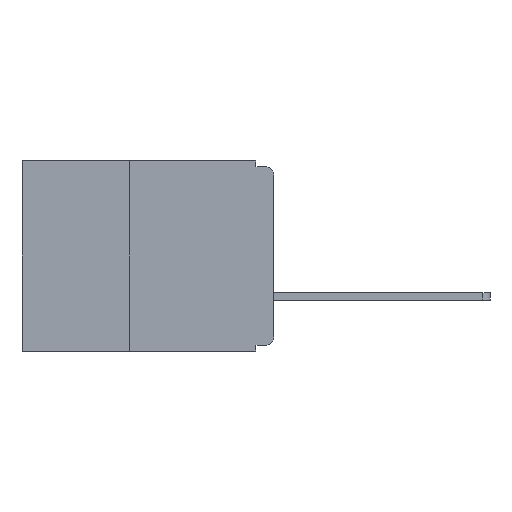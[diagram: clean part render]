
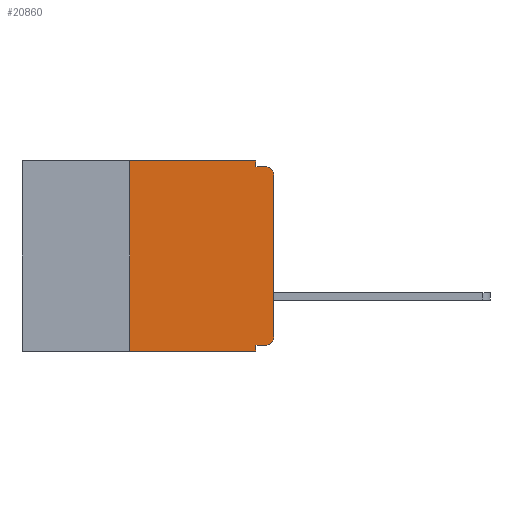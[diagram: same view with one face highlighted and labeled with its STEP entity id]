
A CAD part, left-side view. The second image highlights one B-rep face of the part: STEP entity #20860.
In plain terms, the highlighted planar face has unit normal (-1, 0, 0).
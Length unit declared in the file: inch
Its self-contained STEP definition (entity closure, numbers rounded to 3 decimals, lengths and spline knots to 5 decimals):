
#31 = CIRCLE ( 'NONE', #7282, 0.015 ) ;
#987 = VECTOR ( 'NONE', #13151, 39.37008 ) ;
#1114 = ORIENTED_EDGE ( 'NONE', *, *, #11044, .F. ) ;
#1676 = VECTOR ( 'NONE', #19482, 39.37008 ) ;
#2012 = CARTESIAN_POINT ( 'NONE',  ( 0., 0.437, 0. ) ) ;
#2545 = EDGE_CURVE ( 'NONE', #19357, #19807, #5549, .T. ) ;
#2697 = CARTESIAN_POINT ( 'NONE',  ( 0., 0.25, -0.33 ) ) ;
#3105 = CARTESIAN_POINT ( 'NONE',  ( 0., 0.437, -0.33 ) ) ;
#3606 = VECTOR ( 'NONE', #7558, 39.37008 ) ;
#3786 = VECTOR ( 'NONE', #6497, 39.37008 ) ;
#3992 = DIRECTION ( 'NONE',  ( 0., 0., -1. ) ) ;
#4213 = ORIENTED_EDGE ( 'NONE', *, *, #23866, .T. ) ;
#4277 = CARTESIAN_POINT ( 'NONE',  ( 0., 0.031, -0.33 ) ) ;
#4579 = VERTEX_POINT ( 'NONE', #4277 ) ;
#5303 = EDGE_CURVE ( 'NONE', #5552, #5489, #23249, .T. ) ;
#5489 = VERTEX_POINT ( 'NONE', #20240 ) ;
#5549 = LINE ( 'NONE', #13090, #987 ) ;
#5552 = VERTEX_POINT ( 'NONE', #15027 ) ;
#5753 = VECTOR ( 'NONE', #14703, 39.37008 ) ;
#6497 = DIRECTION ( 'NONE',  ( 0., 0., 1. ) ) ;
#6814 = CARTESIAN_POINT ( 'NONE',  ( 0., 0., -0.32 ) ) ;
#7050 = VECTOR ( 'NONE', #13573, 39.37008 ) ;
#7282 = AXIS2_PLACEMENT_3D ( 'NONE', #11602, #24507, #13502 ) ;
#7558 = DIRECTION ( 'NONE',  ( 0., 0., -1. ) ) ;
#8058 = EDGE_CURVE ( 'NONE', #11526, #17734, #8220, .T. ) ;
#8128 = EDGE_CURVE ( 'NONE', #5552, #4579, #11555, .T. ) ;
#8156 = ORIENTED_EDGE ( 'NONE', *, *, #8128, .T. ) ;
#8220 = LINE ( 'NONE', #6814, #17069 ) ;
#9591 = VERTEX_POINT ( 'NONE', #24304 ) ;
#9617 = EDGE_CURVE ( 'NONE', #17734, #4579, #19310, .T. ) ;
#10279 = VERTEX_POINT ( 'NONE', #24514 ) ;
#10281 = ORIENTED_EDGE ( 'NONE', *, *, #17128, .T. ) ;
#10632 = FACE_OUTER_BOUND ( 'NONE', #12811, .T. ) ;
#11044 = EDGE_CURVE ( 'NONE', #19807, #9591, #16958, .T. ) ;
#11526 = VERTEX_POINT ( 'NONE', #24456 ) ;
#11544 = CARTESIAN_POINT ( 'NONE',  ( 0., 0.015, -0.025 ) ) ;
#11555 = LINE ( 'NONE', #3105, #5753 ) ;
#11602 = CARTESIAN_POINT ( 'NONE',  ( 0., 0.015, -0.305 ) ) ;
#12089 = ORIENTED_EDGE ( 'NONE', *, *, #2545, .F. ) ;
#12672 = ORIENTED_EDGE ( 'NONE', *, *, #5303, .F. ) ;
#12811 = EDGE_LOOP ( 'NONE', ( #10281, #15853, #1114, #12089, #21926, #12672, #8156, #18140, #18718, #4213 ) ) ;
#13090 = CARTESIAN_POINT ( 'NONE',  ( 0., 0.031, 0. ) ) ;
#13151 = DIRECTION ( 'NONE',  ( 0., 0., -1. ) ) ;
#13290 = CARTESIAN_POINT ( 'NONE',  ( 0., 0.031, -0.33 ) ) ;
#13433 = DIRECTION ( 'NONE',  ( 0., 0., -1. ) ) ;
#13502 = DIRECTION ( 'NONE',  ( 0., 0., -1. ) ) ;
#13573 = DIRECTION ( 'NONE',  ( 0., 0., 1. ) ) ;
#13769 = DIRECTION ( 'NONE',  ( 0., -1., 0. ) ) ;
#14703 = DIRECTION ( 'NONE',  ( 0., -1., 0. ) ) ;
#14949 = VECTOR ( 'NONE', #13769, 39.37008 ) ;
#15027 = CARTESIAN_POINT ( 'NONE',  ( 0., 0.25, -0.33 ) ) ;
#15225 = CIRCLE ( 'NONE', #16422, 0.015 ) ;
#15451 = DIRECTION ( 'NONE',  ( 1., 0., 0. ) ) ;
#15521 = LINE ( 'NONE', #22953, #14949 ) ;
#15830 = CARTESIAN_POINT ( 'NONE',  ( 0., 0., -0.025 ) ) ;
#15853 = ORIENTED_EDGE ( 'NONE', *, *, #17816, .T. ) ;
#16422 = AXIS2_PLACEMENT_3D ( 'NONE', #11544, #24438, #13433 ) ;
#16958 = LINE ( 'NONE', #17653, #1676 ) ;
#17069 = VECTOR ( 'NONE', #23687, 39.37008 ) ;
#17128 = EDGE_CURVE ( 'NONE', #10279, #23320, #17699, .T. ) ;
#17234 = CARTESIAN_POINT ( 'NONE',  ( 0., 0.031, -0.32 ) ) ;
#17653 = CARTESIAN_POINT ( 'NONE',  ( 0., 0., -0.01 ) ) ;
#17699 = LINE ( 'NONE', #22754, #7050 ) ;
#17734 = VERTEX_POINT ( 'NONE', #17234 ) ;
#17816 = EDGE_CURVE ( 'NONE', #23320, #9591, #15225, .T. ) ;
#17918 = CARTESIAN_POINT ( 'NONE',  ( 0., 0.031, -0.01 ) ) ;
#18140 = ORIENTED_EDGE ( 'NONE', *, *, #9617, .F. ) ;
#18718 = ORIENTED_EDGE ( 'NONE', *, *, #8058, .F. ) ;
#19310 = LINE ( 'NONE', #13290, #3606 ) ;
#19357 = VERTEX_POINT ( 'NONE', #20106 ) ;
#19482 = DIRECTION ( 'NONE',  ( 0., -1., 0. ) ) ;
#19807 = VERTEX_POINT ( 'NONE', #17918 ) ;
#20106 = CARTESIAN_POINT ( 'NONE',  ( 0., 0.031, 0. ) ) ;
#20240 = CARTESIAN_POINT ( 'NONE',  ( 0., 0.25, 0. ) ) ;
#20860 = ADVANCED_FACE ( 'NONE', ( #10632 ), #22795, .F. ) ;
#21263 = AXIS2_PLACEMENT_3D ( 'NONE', #2012, #15451, #3992 ) ;
#21926 = ORIENTED_EDGE ( 'NONE', *, *, #22612, .F. ) ;
#22612 = EDGE_CURVE ( 'NONE', #5489, #19357, #15521, .T. ) ;
#22754 = CARTESIAN_POINT ( 'NONE',  ( 0., 0., 0. ) ) ;
#22795 = PLANE ( 'NONE',  #21263 ) ;
#22953 = CARTESIAN_POINT ( 'NONE',  ( 0., 0.437, 0. ) ) ;
#23249 = LINE ( 'NONE', #2697, #3786 ) ;
#23320 = VERTEX_POINT ( 'NONE', #15830 ) ;
#23687 = DIRECTION ( 'NONE',  ( 0., 1., 0. ) ) ;
#23866 = EDGE_CURVE ( 'NONE', #11526, #10279, #31, .T. ) ;
#24304 = CARTESIAN_POINT ( 'NONE',  ( 0., 0.015, -0.01 ) ) ;
#24438 = DIRECTION ( 'NONE',  ( -1., 0., 0. ) ) ;
#24456 = CARTESIAN_POINT ( 'NONE',  ( 0., 0.015, -0.32 ) ) ;
#24507 = DIRECTION ( 'NONE',  ( -1., 0., 0. ) ) ;
#24514 = CARTESIAN_POINT ( 'NONE',  ( 0., 0., -0.305 ) ) ;
